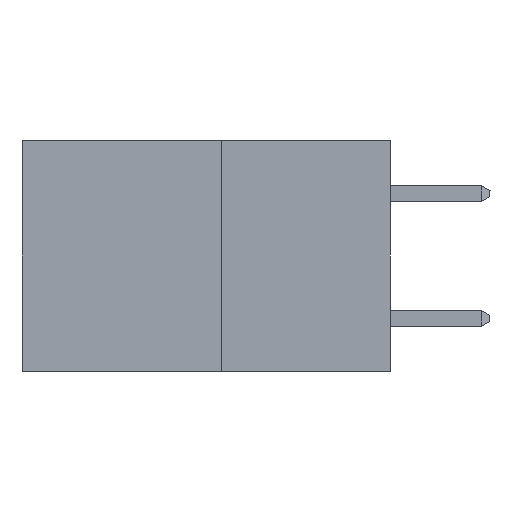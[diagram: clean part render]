
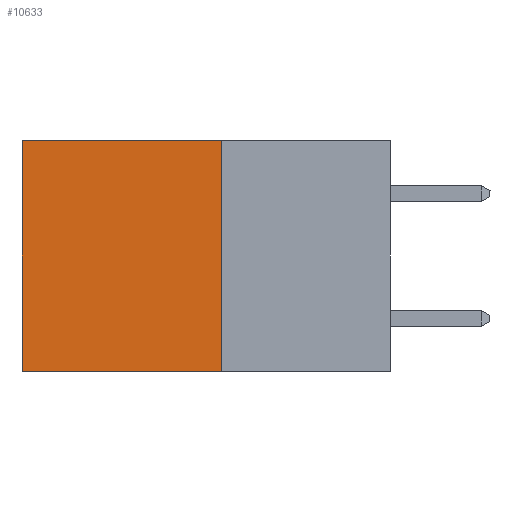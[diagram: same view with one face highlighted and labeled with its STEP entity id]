
A CAD part, left-side view. The second image highlights one B-rep face of the part: STEP entity #10633.
In plain terms, the highlighted planar face has unit normal (-1, 0, 0).
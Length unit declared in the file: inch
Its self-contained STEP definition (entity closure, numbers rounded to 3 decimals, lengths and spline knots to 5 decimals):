
#95 = EDGE_CURVE ( 'NONE', #525, #10318, #14648, .T. ) ;
#525 = VERTEX_POINT ( 'NONE', #18855 ) ;
#538 = DIRECTION ( 'NONE',  ( 0., 1., 0. ) ) ;
#616 = CARTESIAN_POINT ( 'NONE',  ( 0.277, 0.27, -0.37 ) ) ;
#1185 = EDGE_LOOP ( 'NONE', ( #12270, #15957, #8708, #5156 ) ) ;
#1889 = VECTOR ( 'NONE', #14620, 39.37008 ) ;
#1900 = LINE ( 'NONE', #5926, #6147 ) ;
#1960 = VECTOR ( 'NONE', #538, 39.37008 ) ;
#3715 = DIRECTION ( 'NONE',  ( 1., 0., 0. ) ) ;
#5156 = ORIENTED_EDGE ( 'NONE', *, *, #95, .T. ) ;
#5926 = CARTESIAN_POINT ( 'NONE',  ( 0.277, 0.27, -0.37 ) ) ;
#5979 = FACE_OUTER_BOUND ( 'NONE', #1185, .T. ) ;
#6074 = CARTESIAN_POINT ( 'NONE',  ( 0.277, 0.59, 0. ) ) ;
#6147 = VECTOR ( 'NONE', #18482, 39.37008 ) ;
#6455 = CARTESIAN_POINT ( 'NONE',  ( 0.277, 0.27, 0. ) ) ;
#7655 = EDGE_CURVE ( 'NONE', #10318, #12372, #9800, .T. ) ;
#8422 = CARTESIAN_POINT ( 'NONE',  ( 0.277, 0.27, -0.37 ) ) ;
#8708 = ORIENTED_EDGE ( 'NONE', *, *, #12383, .F. ) ;
#9095 = AXIS2_PLACEMENT_3D ( 'NONE', #8422, #3715, #14803 ) ;
#9800 = LINE ( 'NONE', #17545, #17662 ) ;
#10063 = VERTEX_POINT ( 'NONE', #616 ) ;
#10318 = VERTEX_POINT ( 'NONE', #6074 ) ;
#10633 = ADVANCED_FACE ( 'NONE', ( #5979 ), #11644, .F. ) ;
#11644 = PLANE ( 'NONE',  #9095 ) ;
#12270 = ORIENTED_EDGE ( 'NONE', *, *, #7655, .T. ) ;
#12372 = VERTEX_POINT ( 'NONE', #15390 ) ;
#12383 = EDGE_CURVE ( 'NONE', #525, #10063, #1900, .T. ) ;
#13114 = CARTESIAN_POINT ( 'NONE',  ( 0.277, 0.27, -0.37 ) ) ;
#14499 = DIRECTION ( 'NONE',  ( 0., 0., -1. ) ) ;
#14620 = DIRECTION ( 'NONE',  ( 0., 1., 0. ) ) ;
#14648 = LINE ( 'NONE', #6455, #1960 ) ;
#14803 = DIRECTION ( 'NONE',  ( 0., 0., -1. ) ) ;
#15390 = CARTESIAN_POINT ( 'NONE',  ( 0.277, 0.59, -0.37 ) ) ;
#15957 = ORIENTED_EDGE ( 'NONE', *, *, #17068, .F. ) ;
#17068 = EDGE_CURVE ( 'NONE', #10063, #12372, #18180, .T. ) ;
#17545 = CARTESIAN_POINT ( 'NONE',  ( 0.277, 0.59, -0.37 ) ) ;
#17662 = VECTOR ( 'NONE', #14499, 39.37008 ) ;
#18180 = LINE ( 'NONE', #13114, #1889 ) ;
#18482 = DIRECTION ( 'NONE',  ( 0., 0., -1. ) ) ;
#18855 = CARTESIAN_POINT ( 'NONE',  ( 0.277, 0.27, 0. ) ) ;
